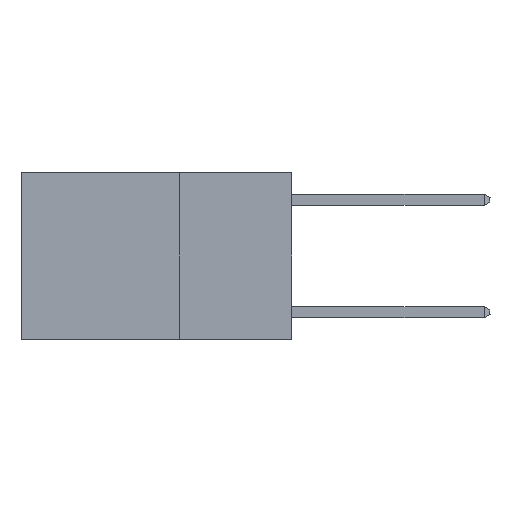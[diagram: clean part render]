
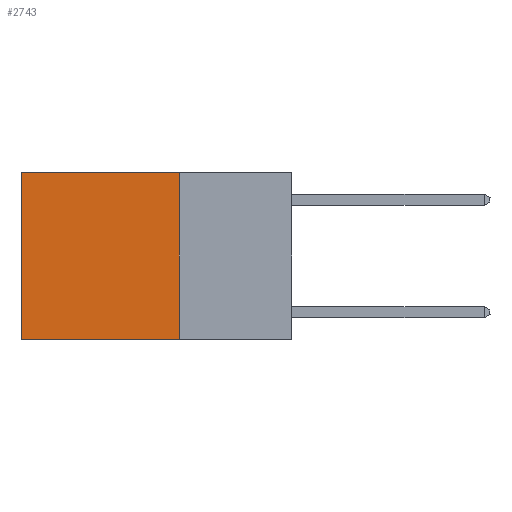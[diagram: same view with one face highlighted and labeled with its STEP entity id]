
A CAD part, left-side view. The second image highlights one B-rep face of the part: STEP entity #2743.
In plain terms, the highlighted planar face has unit normal (-1, 0, 0).
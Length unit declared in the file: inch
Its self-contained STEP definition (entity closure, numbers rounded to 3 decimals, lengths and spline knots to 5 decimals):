
#1921 = CARTESIAN_POINT ( 'NONE',  ( 0.2625, 0.25, 0. ) ) ;
#2383 = ORIENTED_EDGE ( 'NONE', *, *, #24027, .T. ) ;
#2687 = EDGE_CURVE ( 'NONE', #22632, #6112, #9446, .T. ) ;
#2743 = ADVANCED_FACE ( 'NONE', ( #14049 ), #19909, .F. ) ;
#5520 = DIRECTION ( 'NONE',  ( 0., 0., -1. ) ) ;
#5804 = ORIENTED_EDGE ( 'NONE', *, *, #17457, .F. ) ;
#6052 = VERTEX_POINT ( 'NONE', #13194 ) ;
#6112 = VERTEX_POINT ( 'NONE', #22906 ) ;
#6413 = ORIENTED_EDGE ( 'NONE', *, *, #2687, .F. ) ;
#7600 = CARTESIAN_POINT ( 'NONE',  ( 0.2625, 0.6, 0. ) ) ;
#8089 = VECTOR ( 'NONE', #11465, 39.37008 ) ;
#8528 = DIRECTION ( 'NONE',  ( 1., 0., 0. ) ) ;
#9025 = CARTESIAN_POINT ( 'NONE',  ( 0.2625, 0.25, -0.37 ) ) ;
#9446 = LINE ( 'NONE', #20967, #19414 ) ;
#10200 = DIRECTION ( 'NONE',  ( 0., 0., -1. ) ) ;
#10838 = AXIS2_PLACEMENT_3D ( 'NONE', #18139, #8528, #10200 ) ;
#11004 = ORIENTED_EDGE ( 'NONE', *, *, #20969, .T. ) ;
#11315 = DIRECTION ( 'NONE',  ( 0., 1., 0. ) ) ;
#11441 = EDGE_LOOP ( 'NONE', ( #2383, #6413, #5804, #11004 ) ) ;
#11465 = DIRECTION ( 'NONE',  ( 0., 0., -1. ) ) ;
#12305 = CARTESIAN_POINT ( 'NONE',  ( 0.2625, 0.25, 0. ) ) ;
#13194 = CARTESIAN_POINT ( 'NONE',  ( 0.2625, 0.6, 0. ) ) ;
#13718 = VECTOR ( 'NONE', #11315, 39.37008 ) ;
#14049 = FACE_OUTER_BOUND ( 'NONE', #11441, .T. ) ;
#14681 = LINE ( 'NONE', #1921, #24286 ) ;
#17266 = DIRECTION ( 'NONE',  ( 0., 1., 0. ) ) ;
#17457 = EDGE_CURVE ( 'NONE', #17626, #22632, #14681, .T. ) ;
#17626 = VERTEX_POINT ( 'NONE', #12305 ) ;
#18139 = CARTESIAN_POINT ( 'NONE',  ( 0.2625, 0.25, 0. ) ) ;
#19141 = LINE ( 'NONE', #7600, #8089 ) ;
#19414 = VECTOR ( 'NONE', #17266, 39.37008 ) ;
#19909 = PLANE ( 'NONE',  #10838 ) ;
#20967 = CARTESIAN_POINT ( 'NONE',  ( 0.2625, 0.25, -0.37 ) ) ;
#20969 = EDGE_CURVE ( 'NONE', #17626, #6052, #21304, .T. ) ;
#21304 = LINE ( 'NONE', #23222, #13718 ) ;
#22632 = VERTEX_POINT ( 'NONE', #9025 ) ;
#22906 = CARTESIAN_POINT ( 'NONE',  ( 0.2625, 0.6, -0.37 ) ) ;
#23222 = CARTESIAN_POINT ( 'NONE',  ( 0.2625, 0.25, 0. ) ) ;
#24027 = EDGE_CURVE ( 'NONE', #6052, #6112, #19141, .T. ) ;
#24286 = VECTOR ( 'NONE', #5520, 39.37008 ) ;
